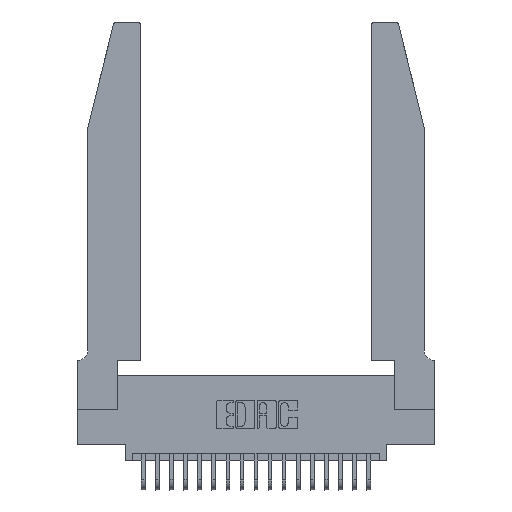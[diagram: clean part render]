
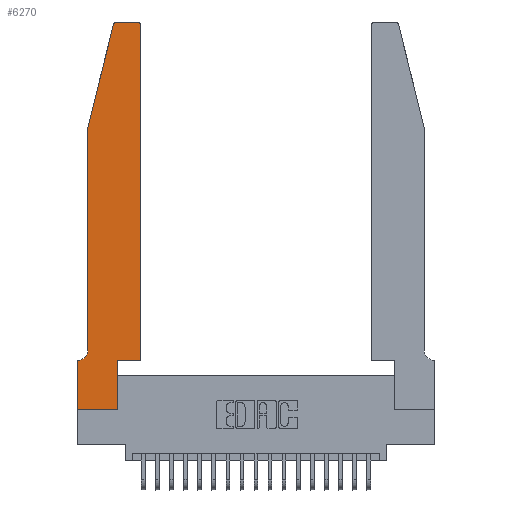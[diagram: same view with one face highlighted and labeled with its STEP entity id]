
A CAD part, top view. The second image highlights one B-rep face of the part: STEP entity #6270.
In plain terms, the highlighted planar face has unit normal (0, 0, 1).
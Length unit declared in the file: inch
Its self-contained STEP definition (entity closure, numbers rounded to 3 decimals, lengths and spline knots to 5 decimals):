
#11 = VECTOR ( 'NONE', #5644, 39.37008 ) ;
#188 = VERTEX_POINT ( 'NONE', #15390 ) ;
#279 = EDGE_CURVE ( 'NONE', #2934, #12175, #9177, .T. ) ;
#584 = VECTOR ( 'NONE', #10148, 39.37008 ) ;
#1295 = VERTEX_POINT ( 'NONE', #6136 ) ;
#1652 = EDGE_CURVE ( 'NONE', #14923, #7414, #11307, .T. ) ;
#2324 = DIRECTION ( 'NONE',  ( 0., 0., -1. ) ) ;
#2509 = LINE ( 'NONE', #2955, #11564 ) ;
#2619 = CARTESIAN_POINT ( 'NONE',  ( 0.4505, 0.35, 0.37 ) ) ;
#2787 = DIRECTION ( 'NONE',  ( 0., 0., 1. ) ) ;
#2934 = VERTEX_POINT ( 'NONE', #21411 ) ;
#2955 = CARTESIAN_POINT ( 'NONE',  ( 0.0755, 0.35, 0.37 ) ) ;
#3010 = AXIS2_PLACEMENT_3D ( 'NONE', #13137, #2324, #14930 ) ;
#3243 = ORIENTED_EDGE ( 'NONE', *, *, #1652, .T. ) ;
#3550 = CARTESIAN_POINT ( 'NONE',  ( 0.4505, 0.35, 0.37 ) ) ;
#4209 = VERTEX_POINT ( 'NONE', #9635 ) ;
#4212 = CIRCLE ( 'NONE', #5042, 0.03 ) ;
#4535 = DIRECTION ( 'NONE',  ( 1., 0., 0. ) ) ;
#4556 = CARTESIAN_POINT ( 'NONE',  ( 0.25487, 2.72718, 0.37 ) ) ;
#4651 = ORIENTED_EDGE ( 'NONE', *, *, #14808, .T. ) ;
#4875 = DIRECTION ( 'NONE',  ( -1., 0., 0. ) ) ;
#5042 = AXIS2_PLACEMENT_3D ( 'NONE', #20174, #9526, #21944 ) ;
#5277 = CARTESIAN_POINT ( 'NONE',  ( 0.0755, 2., 0.37 ) ) ;
#5311 = DIRECTION ( 'NONE',  ( 0., 0., 1. ) ) ;
#5644 = DIRECTION ( 'NONE',  ( 0., 1., 0. ) ) ;
#6136 = CARTESIAN_POINT ( 'NONE',  ( 0.0755, 0.42, 0.37 ) ) ;
#6270 = ADVANCED_FACE ( 'NONE', ( #19077 ), #23012, .T. ) ;
#6607 = VECTOR ( 'NONE', #19622, 39.37008 ) ;
#7414 = VERTEX_POINT ( 'NONE', #19402 ) ;
#7528 = VERTEX_POINT ( 'NONE', #12919 ) ;
#7916 = DIRECTION ( 'NONE',  ( 0., -1., 0. ) ) ;
#8038 = CIRCLE ( 'NONE', #22257, 0.03 ) ;
#8395 = CARTESIAN_POINT ( 'NONE',  ( 0.2605, 2.75, 0.37 ) ) ;
#8718 = CARTESIAN_POINT ( 'NONE',  ( 0.2865, 0., 0.37 ) ) ;
#8955 = AXIS2_PLACEMENT_3D ( 'NONE', #19467, #5311, #17770 ) ;
#9177 = LINE ( 'NONE', #3550, #11 ) ;
#9410 = VECTOR ( 'NONE', #12121, 39.37008 ) ;
#9433 = ORIENTED_EDGE ( 'NONE', *, *, #15888, .T. ) ;
#9526 = DIRECTION ( 'NONE',  ( 0., 0., 1. ) ) ;
#9635 = CARTESIAN_POINT ( 'NONE',  ( 0.0755, 2., 0.37 ) ) ;
#10148 = DIRECTION ( 'NONE',  ( -1., 0., 0. ) ) ;
#10347 = CARTESIAN_POINT ( 'NONE',  ( 0.0755, 2., 0.37 ) ) ;
#10414 = VECTOR ( 'NONE', #23058, 39.37008 ) ;
#11078 = EDGE_CURVE ( 'NONE', #22868, #12845, #15002, .T. ) ;
#11307 = LINE ( 'NONE', #14719, #6607 ) ;
#11459 = ORIENTED_EDGE ( 'NONE', *, *, #16713, .T. ) ;
#11564 = VECTOR ( 'NONE', #4875, 39.37008 ) ;
#11818 = EDGE_CURVE ( 'NONE', #4209, #1295, #18859, .T. ) ;
#12121 = DIRECTION ( 'NONE',  ( 0., -1., 0. ) ) ;
#12175 = VERTEX_POINT ( 'NONE', #17071 ) ;
#12181 = VERTEX_POINT ( 'NONE', #4556 ) ;
#12236 = ORIENTED_EDGE ( 'NONE', *, *, #20031, .T. ) ;
#12432 = LINE ( 'NONE', #16770, #13544 ) ;
#12704 = CIRCLE ( 'NONE', #3010, 0.07 ) ;
#12845 = VERTEX_POINT ( 'NONE', #22420 ) ;
#12919 = CARTESIAN_POINT ( 'NONE',  ( 0., 0., 0.37 ) ) ;
#13012 = CARTESIAN_POINT ( 'NONE',  ( 0.4205, 2.75, 0.37 ) ) ;
#13019 = LINE ( 'NONE', #2619, #21928 ) ;
#13087 = EDGE_CURVE ( 'NONE', #12175, #22868, #8038, .T. ) ;
#13137 = CARTESIAN_POINT ( 'NONE',  ( 0.0055, 0.42, 0.37 ) ) ;
#13517 = EDGE_CURVE ( 'NONE', #13534, #7528, #22157, .T. ) ;
#13534 = VERTEX_POINT ( 'NONE', #20337 ) ;
#13544 = VECTOR ( 'NONE', #16611, 39.37008 ) ;
#13564 = ORIENTED_EDGE ( 'NONE', *, *, #13087, .T. ) ;
#13565 = CARTESIAN_POINT ( 'NONE',  ( 0.4205, 2.72, 0.37 ) ) ;
#14084 = EDGE_CURVE ( 'NONE', #7528, #14923, #12432, .T. ) ;
#14156 = ORIENTED_EDGE ( 'NONE', *, *, #13517, .T. ) ;
#14719 = CARTESIAN_POINT ( 'NONE',  ( 0.2865, 0.35, 0.37 ) ) ;
#14808 = EDGE_CURVE ( 'NONE', #188, #13534, #2509, .T. ) ;
#14923 = VERTEX_POINT ( 'NONE', #8718 ) ;
#14930 = DIRECTION ( 'NONE',  ( -1., 0., 0. ) ) ;
#14960 = CARTESIAN_POINT ( 'NONE',  ( 0., 0., 0.37 ) ) ;
#15002 = LINE ( 'NONE', #8395, #584 ) ;
#15157 = LINE ( 'NONE', #5277, #10414 ) ;
#15386 = DIRECTION ( 'NONE',  ( 1., 0., 0. ) ) ;
#15390 = CARTESIAN_POINT ( 'NONE',  ( 0.0055, 0.35, 0.37 ) ) ;
#15888 = EDGE_CURVE ( 'NONE', #12181, #4209, #15157, .T. ) ;
#16611 = DIRECTION ( 'NONE',  ( 1., 0., 0. ) ) ;
#16713 = EDGE_CURVE ( 'NONE', #12845, #12181, #4212, .T. ) ;
#16741 = ORIENTED_EDGE ( 'NONE', *, *, #21326, .T. ) ;
#16770 = CARTESIAN_POINT ( 'NONE',  ( 0., 0., 0.37 ) ) ;
#16998 = ORIENTED_EDGE ( 'NONE', *, *, #279, .T. ) ;
#17071 = CARTESIAN_POINT ( 'NONE',  ( 0.4505, 2.72, 0.37 ) ) ;
#17477 = VECTOR ( 'NONE', #7916, 39.37008 ) ;
#17770 = DIRECTION ( 'NONE',  ( 1., 0., 0. ) ) ;
#18113 = EDGE_LOOP ( 'NONE', ( #21148, #11459, #9433, #20750, #16741, #4651, #14156, #22077, #3243, #12236, #16998, #13564 ) ) ;
#18859 = LINE ( 'NONE', #10347, #9410 ) ;
#19077 = FACE_OUTER_BOUND ( 'NONE', #18113, .T. ) ;
#19402 = CARTESIAN_POINT ( 'NONE',  ( 0.2865, 0.35, 0.37 ) ) ;
#19467 = CARTESIAN_POINT ( 'NONE',  ( 0., 0.35, 0.37 ) ) ;
#19622 = DIRECTION ( 'NONE',  ( 0., 1., 0. ) ) ;
#20031 = EDGE_CURVE ( 'NONE', #7414, #2934, #13019, .T. ) ;
#20174 = CARTESIAN_POINT ( 'NONE',  ( 0.284, 2.72, 0.37 ) ) ;
#20337 = CARTESIAN_POINT ( 'NONE',  ( 0., 0.35, 0.37 ) ) ;
#20750 = ORIENTED_EDGE ( 'NONE', *, *, #11818, .T. ) ;
#21148 = ORIENTED_EDGE ( 'NONE', *, *, #11078, .T. ) ;
#21326 = EDGE_CURVE ( 'NONE', #1295, #188, #12704, .T. ) ;
#21411 = CARTESIAN_POINT ( 'NONE',  ( 0.4505, 0.35, 0.37 ) ) ;
#21928 = VECTOR ( 'NONE', #4535, 39.37008 ) ;
#21944 = DIRECTION ( 'NONE',  ( 1., 0., 0. ) ) ;
#22077 = ORIENTED_EDGE ( 'NONE', *, *, #14084, .T. ) ;
#22157 = LINE ( 'NONE', #14960, #17477 ) ;
#22257 = AXIS2_PLACEMENT_3D ( 'NONE', #13565, #2787, #15386 ) ;
#22420 = CARTESIAN_POINT ( 'NONE',  ( 0.284, 2.75, 0.37 ) ) ;
#22868 = VERTEX_POINT ( 'NONE', #13012 ) ;
#23012 = PLANE ( 'NONE',  #8955 ) ;
#23058 = DIRECTION ( 'NONE',  ( -0.239, -0.971, 0. ) ) ;
